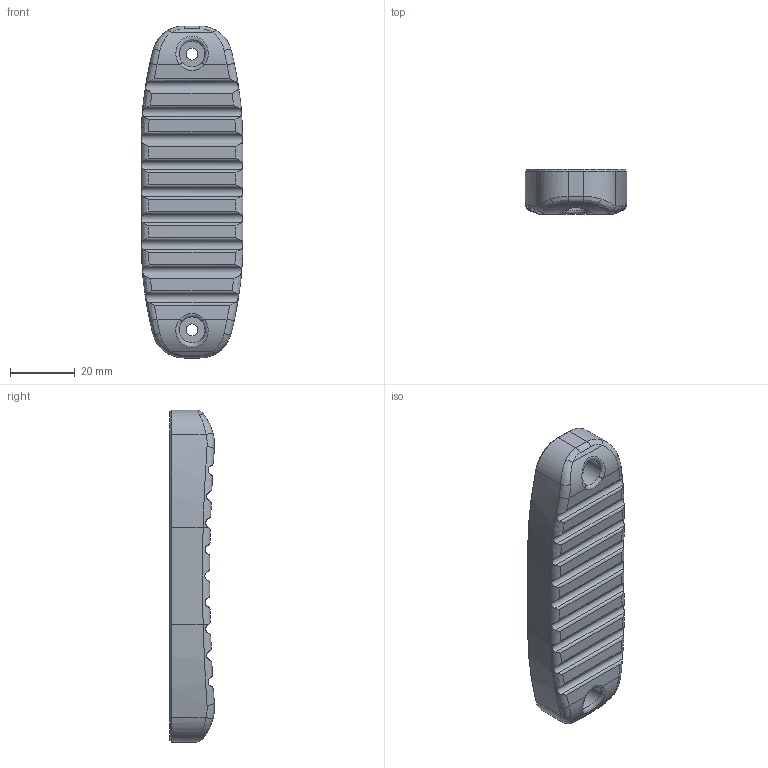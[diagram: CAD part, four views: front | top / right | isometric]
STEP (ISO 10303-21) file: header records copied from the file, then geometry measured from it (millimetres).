
FILE_DESCRIPTION(/* description */ (''),/* implementation_level */ '2;1');
FILE_NAME(/* name */ 'Concave Buttpad.step',/* time_stamp */ '2021-09-27T04:49:37-04:00',/* author */ (''),/* organization */ (''),/* preprocessor_version */ 'ST-DEVELOPER v18.1',/* originating_system */ 'Autodesk Translation Framework v10.10.0.1391',/* authorisation */ '');
FILE_SCHEMA (('AUTOMOTIVE_DESIGN { 1 0 10303 214 3 1 1 }'));
Length unit declared in the file: millimetre
Products named in the file (1): Concave Buttstock
Bounding box: 31.5 x 13.86 x 102.57 mm (x, y, z)
Volume: 25825.3 mm3; surface area: 10327.4 mm2
Topology: 1 solids, 1 shells, 182 faces, 438 edges, 252 vertices
Faces by surface type: cylinder 79, bspline 28, plane 27, torus 24, cone 24
Full cylindrical faces by diameter (mm): 3.7 x2, 8 x2
Entity records: 7020 total; most frequent: CARTESIAN_POINT 2987, ORIENTED_EDGE 860, DIRECTION 800, EDGE_CURVE 430, AXIS2_PLACEMENT_3D 323, VERTEX_POINT 252, EDGE_LOOP 188, FACE_OUTER_BOUND 182
